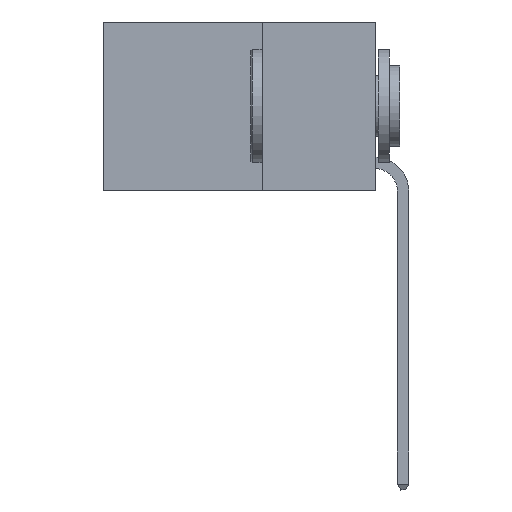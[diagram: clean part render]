
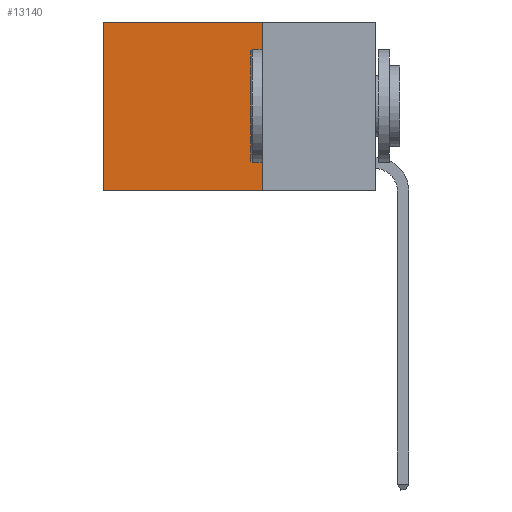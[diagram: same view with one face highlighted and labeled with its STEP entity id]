
A CAD part, left-side view. The second image highlights one B-rep face of the part: STEP entity #13140.
In plain terms, the highlighted planar face has unit normal (-1, 0, 0).
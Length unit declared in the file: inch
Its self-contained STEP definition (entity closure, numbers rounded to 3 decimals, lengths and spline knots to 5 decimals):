
#713 = CARTESIAN_POINT ( 'NONE',  ( 0.2625, 0.6, 0. ) ) ;
#771 = ORIENTED_EDGE ( 'NONE', *, *, #4100, .T. ) ;
#3953 = VERTEX_POINT ( 'NONE', #5411 ) ;
#4100 = EDGE_CURVE ( 'NONE', #15661, #9986, #12088, .T. ) ;
#4705 = VERTEX_POINT ( 'NONE', #8026 ) ;
#5411 = CARTESIAN_POINT ( 'NONE',  ( 0.2625, 0.25, 0. ) ) ;
#6237 = LINE ( 'NONE', #11295, #7403 ) ;
#6335 = CARTESIAN_POINT ( 'NONE',  ( 0.2625, 0.25, 0. ) ) ;
#7403 = VECTOR ( 'NONE', #15105, 39.37008 ) ;
#8026 = CARTESIAN_POINT ( 'NONE',  ( 0.2625, 0.25, -0.37 ) ) ;
#8198 = ORIENTED_EDGE ( 'NONE', *, *, #9208, .F. ) ;
#8853 = VECTOR ( 'NONE', #13468, 39.37008 ) ;
#9118 = ORIENTED_EDGE ( 'NONE', *, *, #9188, .F. ) ;
#9188 = EDGE_CURVE ( 'NONE', #4705, #9986, #9730, .T. ) ;
#9208 = EDGE_CURVE ( 'NONE', #3953, #4705, #11946, .T. ) ;
#9478 = CARTESIAN_POINT ( 'NONE',  ( 0.2625, 0.6, 0. ) ) ;
#9492 = CARTESIAN_POINT ( 'NONE',  ( 0.2625, 0.25, -0.37 ) ) ;
#9730 = LINE ( 'NONE', #9492, #15869 ) ;
#9986 = VERTEX_POINT ( 'NONE', #10499 ) ;
#10007 = PLANE ( 'NONE',  #14869 ) ;
#10499 = CARTESIAN_POINT ( 'NONE',  ( 0.2625, 0.6, -0.37 ) ) ;
#10873 = CARTESIAN_POINT ( 'NONE',  ( 0.2625, 0.25, 0. ) ) ;
#11227 = FACE_OUTER_BOUND ( 'NONE', #15947, .T. ) ;
#11295 = CARTESIAN_POINT ( 'NONE',  ( 0.2625, 0.25, 0. ) ) ;
#11946 = LINE ( 'NONE', #10873, #8853 ) ;
#12088 = LINE ( 'NONE', #713, #13104 ) ;
#13104 = VECTOR ( 'NONE', #14514, 39.37008 ) ;
#13140 = ADVANCED_FACE ( 'NONE', ( #11227 ), #10007, .F. ) ;
#13468 = DIRECTION ( 'NONE',  ( 0., 0., -1. ) ) ;
#13889 = DIRECTION ( 'NONE',  ( 1., 0., 0. ) ) ;
#14514 = DIRECTION ( 'NONE',  ( 0., 0., -1. ) ) ;
#14528 = DIRECTION ( 'NONE',  ( 0., 1., 0. ) ) ;
#14869 = AXIS2_PLACEMENT_3D ( 'NONE', #6335, #13889, #15043 ) ;
#14922 = EDGE_CURVE ( 'NONE', #3953, #15661, #6237, .T. ) ;
#15043 = DIRECTION ( 'NONE',  ( 0., 0., -1. ) ) ;
#15105 = DIRECTION ( 'NONE',  ( 0., 1., 0. ) ) ;
#15661 = VERTEX_POINT ( 'NONE', #9478 ) ;
#15869 = VECTOR ( 'NONE', #14528, 39.37008 ) ;
#15870 = ORIENTED_EDGE ( 'NONE', *, *, #14922, .T. ) ;
#15947 = EDGE_LOOP ( 'NONE', ( #771, #9118, #8198, #15870 ) ) ;
